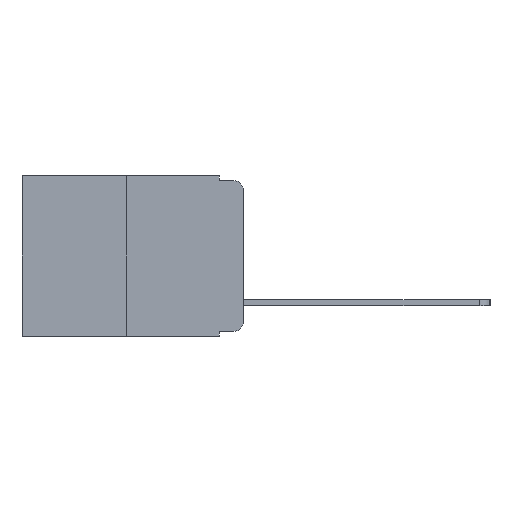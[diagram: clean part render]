
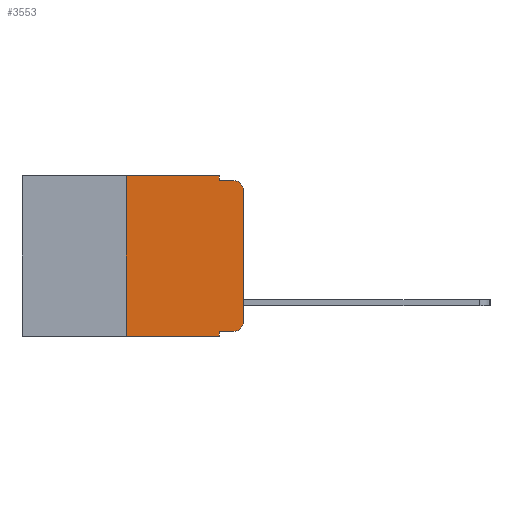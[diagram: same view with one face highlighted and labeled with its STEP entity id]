
A CAD part, left-side view. The second image highlights one B-rep face of the part: STEP entity #3553.
In plain terms, the highlighted planar face has unit normal (-1, 0, 0).
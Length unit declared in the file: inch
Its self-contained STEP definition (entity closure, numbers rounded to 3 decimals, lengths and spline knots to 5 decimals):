
#8 = ORIENTED_EDGE ( 'NONE', *, *, #6719, .T. ) ;
#282 = DIRECTION ( 'NONE',  ( -1., 0., 0. ) ) ;
#383 = AXIS2_PLACEMENT_3D ( 'NONE', #5554, #17726, #7362 ) ;
#2181 = CARTESIAN_POINT ( 'NONE',  ( 0., 0.473, 0. ) ) ;
#2413 = DIRECTION ( 'NONE',  ( 0., -1., 0. ) ) ;
#2559 = VECTOR ( 'NONE', #20003, 39.37008 ) ;
#2923 = ORIENTED_EDGE ( 'NONE', *, *, #6906, .T. ) ;
#3202 = LINE ( 'NONE', #18355, #2559 ) ;
#3229 = ORIENTED_EDGE ( 'NONE', *, *, #6799, .F. ) ;
#3553 = ADVANCED_FACE ( 'NONE', ( #8370 ), #12944, .F. ) ;
#3646 = VERTEX_POINT ( 'NONE', #17000 ) ;
#3820 = CARTESIAN_POINT ( 'NONE',  ( 0., 0., -0.313 ) ) ;
#3955 = VERTEX_POINT ( 'NONE', #16243 ) ;
#4190 = DIRECTION ( 'NONE',  ( 0., 0., -1. ) ) ;
#4363 = EDGE_CURVE ( 'NONE', #15662, #3955, #8076, .T. ) ;
#4712 = CARTESIAN_POINT ( 'NONE',  ( 0., 0.051, -0.333 ) ) ;
#4728 = EDGE_CURVE ( 'NONE', #21283, #17361, #18865, .T. ) ;
#4752 = CARTESIAN_POINT ( 'NONE',  ( 0., 0.02, -0.333 ) ) ;
#5504 = CARTESIAN_POINT ( 'NONE',  ( 0., 0.25, 0. ) ) ;
#5554 = CARTESIAN_POINT ( 'NONE',  ( 0., 0.02, -0.313 ) ) ;
#6143 = CARTESIAN_POINT ( 'NONE',  ( 0., 0.051, 0. ) ) ;
#6271 = DIRECTION ( 'NONE',  ( 0., 0., 1. ) ) ;
#6307 = EDGE_LOOP ( 'NONE', ( #8, #21166, #13194, #18334, #19131, #3229, #8664, #18356, #2923, #21979 ) ) ;
#6418 = CARTESIAN_POINT ( 'NONE',  ( 0., 0.051, 0. ) ) ;
#6500 = DIRECTION ( 'NONE',  ( 0., -1., 0. ) ) ;
#6719 = EDGE_CURVE ( 'NONE', #13020, #3646, #18337, .T. ) ;
#6725 = EDGE_CURVE ( 'NONE', #3646, #10811, #22215, .T. ) ;
#6758 = EDGE_CURVE ( 'NONE', #21521, #10811, #17237, .T. ) ;
#6767 = EDGE_CURVE ( 'NONE', #17361, #21521, #3202, .T. ) ;
#6799 = EDGE_CURVE ( 'NONE', #15662, #21283, #11595, .T. ) ;
#6867 = EDGE_CURVE ( 'NONE', #18009, #3955, #10511, .T. ) ;
#6906 = EDGE_CURVE ( 'NONE', #18009, #14694, #13999, .T. ) ;
#7186 = EDGE_CURVE ( 'NONE', #14694, #13020, #17766, .T. ) ;
#7362 = DIRECTION ( 'NONE',  ( 0., 0., -1. ) ) ;
#7494 = VECTOR ( 'NONE', #19228, 39.37008 ) ;
#7524 = CARTESIAN_POINT ( 'NONE',  ( 0., 0.473, 0. ) ) ;
#8076 = LINE ( 'NONE', #10669, #7494 ) ;
#8245 = DIRECTION ( 'NONE',  ( 0., 0., -1. ) ) ;
#8370 = FACE_OUTER_BOUND ( 'NONE', #6307, .T. ) ;
#8664 = ORIENTED_EDGE ( 'NONE', *, *, #4363, .T. ) ;
#8904 = CARTESIAN_POINT ( 'NONE',  ( 0., 0.25, -0.343 ) ) ;
#9442 = VECTOR ( 'NONE', #6500, 39.37008 ) ;
#9482 = DIRECTION ( 'NONE',  ( 0., 0., 1. ) ) ;
#9639 = CARTESIAN_POINT ( 'NONE',  ( 0., 0.051, -0.01 ) ) ;
#9720 = VECTOR ( 'NONE', #17889, 39.37008 ) ;
#10511 = LINE ( 'NONE', #6418, #14504 ) ;
#10669 = CARTESIAN_POINT ( 'NONE',  ( 0., 0.473, -0.343 ) ) ;
#10811 = VERTEX_POINT ( 'NONE', #21295 ) ;
#11359 = CARTESIAN_POINT ( 'NONE',  ( 0., 0.02, -0.03 ) ) ;
#11595 = LINE ( 'NONE', #18421, #20128 ) ;
#12043 = CARTESIAN_POINT ( 'NONE',  ( 0., 0.051, -0.333 ) ) ;
#12654 = VECTOR ( 'NONE', #2413, 39.37008 ) ;
#12944 = PLANE ( 'NONE',  #17389 ) ;
#12991 = CARTESIAN_POINT ( 'NONE',  ( 0., 0., 0. ) ) ;
#13020 = VERTEX_POINT ( 'NONE', #3820 ) ;
#13061 = DIRECTION ( 'NONE',  ( 0., 0., -1. ) ) ;
#13194 = ORIENTED_EDGE ( 'NONE', *, *, #6758, .F. ) ;
#13999 = LINE ( 'NONE', #4712, #9442 ) ;
#14504 = VECTOR ( 'NONE', #8245, 39.37008 ) ;
#14637 = DIRECTION ( 'NONE',  ( 1., 0., 0. ) ) ;
#14694 = VERTEX_POINT ( 'NONE', #4752 ) ;
#15662 = VERTEX_POINT ( 'NONE', #8904 ) ;
#16243 = CARTESIAN_POINT ( 'NONE',  ( 0., 0.051, -0.343 ) ) ;
#17000 = CARTESIAN_POINT ( 'NONE',  ( 0., 0., -0.03 ) ) ;
#17237 = LINE ( 'NONE', #9639, #12654 ) ;
#17361 = VERTEX_POINT ( 'NONE', #6143 ) ;
#17389 = AXIS2_PLACEMENT_3D ( 'NONE', #2181, #14637, #4190 ) ;
#17726 = DIRECTION ( 'NONE',  ( -1., 0., 0. ) ) ;
#17766 = CIRCLE ( 'NONE', #383, 0.02 ) ;
#17786 = VECTOR ( 'NONE', #9482, 39.37008 ) ;
#17889 = DIRECTION ( 'NONE',  ( 0., -1., 0. ) ) ;
#18009 = VERTEX_POINT ( 'NONE', #12043 ) ;
#18334 = ORIENTED_EDGE ( 'NONE', *, *, #6767, .F. ) ;
#18337 = LINE ( 'NONE', #12991, #17786 ) ;
#18355 = CARTESIAN_POINT ( 'NONE',  ( 0., 0.051, 0. ) ) ;
#18356 = ORIENTED_EDGE ( 'NONE', *, *, #6867, .F. ) ;
#18421 = CARTESIAN_POINT ( 'NONE',  ( 0., 0.25, 0. ) ) ;
#18865 = LINE ( 'NONE', #7524, #9720 ) ;
#19131 = ORIENTED_EDGE ( 'NONE', *, *, #4728, .F. ) ;
#19228 = DIRECTION ( 'NONE',  ( 0., -1., 0. ) ) ;
#20003 = DIRECTION ( 'NONE',  ( 0., 0., -1. ) ) ;
#20128 = VECTOR ( 'NONE', #6271, 39.37008 ) ;
#21166 = ORIENTED_EDGE ( 'NONE', *, *, #6725, .T. ) ;
#21283 = VERTEX_POINT ( 'NONE', #5504 ) ;
#21295 = CARTESIAN_POINT ( 'NONE',  ( 0., 0.02, -0.01 ) ) ;
#21376 = CARTESIAN_POINT ( 'NONE',  ( 0., 0.051, -0.01 ) ) ;
#21471 = AXIS2_PLACEMENT_3D ( 'NONE', #11359, #282, #13061 ) ;
#21521 = VERTEX_POINT ( 'NONE', #21376 ) ;
#21979 = ORIENTED_EDGE ( 'NONE', *, *, #7186, .T. ) ;
#22215 = CIRCLE ( 'NONE', #21471, 0.02 ) ;
